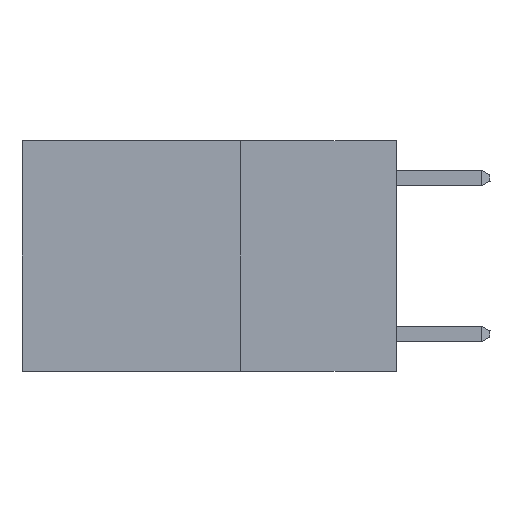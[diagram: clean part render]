
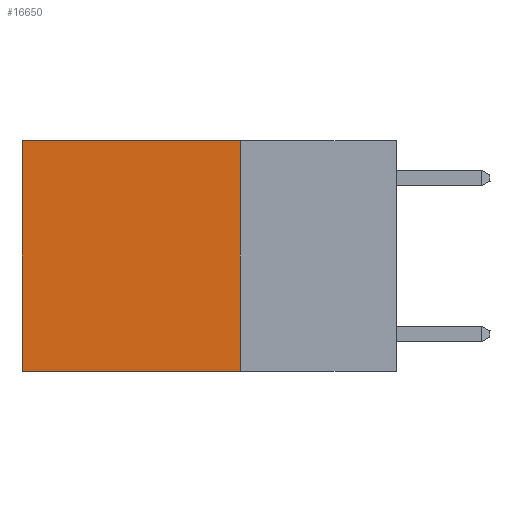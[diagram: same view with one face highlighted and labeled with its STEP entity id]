
A CAD part, left-side view. The second image highlights one B-rep face of the part: STEP entity #16650.
In plain terms, the highlighted planar face has unit normal (-1, 0, 0).
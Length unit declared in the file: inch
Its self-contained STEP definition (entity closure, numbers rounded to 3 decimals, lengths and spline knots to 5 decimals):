
#86 = DIRECTION ( 'NONE',  ( 0., 1., 0. ) ) ;
#762 = EDGE_CURVE ( 'NONE', #11828, #15933, #27616, .T. ) ;
#878 = DIRECTION ( 'NONE',  ( 0., 0., -1. ) ) ;
#2049 = VECTOR ( 'NONE', #8002, 39.37008 ) ;
#4452 = FACE_OUTER_BOUND ( 'NONE', #14285, .T. ) ;
#4681 = VECTOR ( 'NONE', #18475, 39.37008 ) ;
#6381 = CARTESIAN_POINT ( 'NONE',  ( 0.2625, 0.25, 0. ) ) ;
#6455 = VERTEX_POINT ( 'NONE', #6381 ) ;
#8002 = DIRECTION ( 'NONE',  ( 0., 1., 0. ) ) ;
#8552 = DIRECTION ( 'NONE',  ( 1., 0., 0. ) ) ;
#10947 = DIRECTION ( 'NONE',  ( 0., 0., -1. ) ) ;
#10978 = ORIENTED_EDGE ( 'NONE', *, *, #26072, .T. ) ;
#11016 = VECTOR ( 'NONE', #878, 39.37008 ) ;
#11101 = CARTESIAN_POINT ( 'NONE',  ( 0.2625, 0.6, 0. ) ) ;
#11233 = PLANE ( 'NONE',  #15120 ) ;
#11828 = VERTEX_POINT ( 'NONE', #27477 ) ;
#12522 = CARTESIAN_POINT ( 'NONE',  ( 0.2625, 0.25, -0.37 ) ) ;
#12931 = CARTESIAN_POINT ( 'NONE',  ( 0.2625, 0.25, 0. ) ) ;
#14241 = EDGE_CURVE ( 'NONE', #6455, #11828, #18116, .T. ) ;
#14285 = EDGE_LOOP ( 'NONE', ( #17750, #22819, #24833, #10978 ) ) ;
#15120 = AXIS2_PLACEMENT_3D ( 'NONE', #19581, #8552, #10947 ) ;
#15130 = EDGE_CURVE ( 'NONE', #26119, #15933, #19762, .T. ) ;
#15389 = VECTOR ( 'NONE', #86, 39.37008 ) ;
#15586 = CARTESIAN_POINT ( 'NONE',  ( 0.2625, 0.25, 0. ) ) ;
#15933 = VERTEX_POINT ( 'NONE', #27091 ) ;
#16650 = ADVANCED_FACE ( 'NONE', ( #4452 ), #11233, .F. ) ;
#17750 = ORIENTED_EDGE ( 'NONE', *, *, #15130, .T. ) ;
#18054 = CARTESIAN_POINT ( 'NONE',  ( 0.2625, 0.6, 0. ) ) ;
#18116 = LINE ( 'NONE', #15586, #11016 ) ;
#18475 = DIRECTION ( 'NONE',  ( 0., 0., -1. ) ) ;
#19581 = CARTESIAN_POINT ( 'NONE',  ( 0.2625, 0.25, 0. ) ) ;
#19721 = LINE ( 'NONE', #12931, #15389 ) ;
#19762 = LINE ( 'NONE', #18054, #4681 ) ;
#22819 = ORIENTED_EDGE ( 'NONE', *, *, #762, .F. ) ;
#24833 = ORIENTED_EDGE ( 'NONE', *, *, #14241, .F. ) ;
#26072 = EDGE_CURVE ( 'NONE', #6455, #26119, #19721, .T. ) ;
#26119 = VERTEX_POINT ( 'NONE', #11101 ) ;
#27091 = CARTESIAN_POINT ( 'NONE',  ( 0.2625, 0.6, -0.37 ) ) ;
#27477 = CARTESIAN_POINT ( 'NONE',  ( 0.2625, 0.25, -0.37 ) ) ;
#27616 = LINE ( 'NONE', #12522, #2049 ) ;
